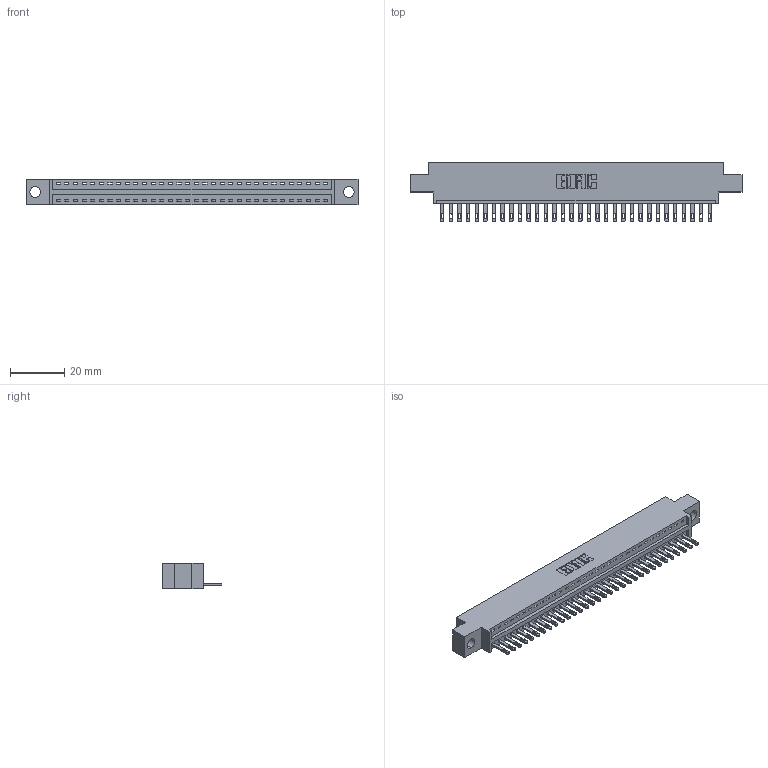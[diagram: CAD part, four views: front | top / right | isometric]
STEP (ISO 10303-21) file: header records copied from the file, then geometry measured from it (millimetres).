
FILE_DESCRIPTION (( 'STEP AP203' ), '1' );
FILE_NAME ('346-032-500-604.STEP', '2022-05-06T17:44:56', ( '' ), ( '' ), 'SwSTEP 2.0', 'SolidWorks 2020', '' );
FILE_SCHEMA (( 'CONFIG_CONTROL_DESIGN' ));
Length unit declared in the file: inch
Products named in the file (3): 346 Part_0.170 Offset - 0.156 Dia-TH; 345-292-001_345-293-100; 346-032-500-604
Assembly tree (33 placements, depth 2):
  346-032-500-604
    346 Part_0.170 Offset - 0.156 Dia-TH
    345-292-001_345-293-100  x32
Bounding box: 122.17 x 21.84 x 9.4 mm (x, y, z)
Volume: 11385.1 mm3; surface area: 14194.2 mm2
Topology: 33 solids, 33 shells, 1868 faces, 5753 edges, 3834 vertices
Faces by surface type: plane 1182, cylinder 686
Entity records: 21687 total; most frequent: CARTESIAN_POINT 3730, ORIENTED_EDGE 3694, DIRECTION 3303, EDGE_CURVE 1847, VECTOR 1583, LINE 1583, VERTEX_POINT 1230, AXIS2_PLACEMENT_3D 860
